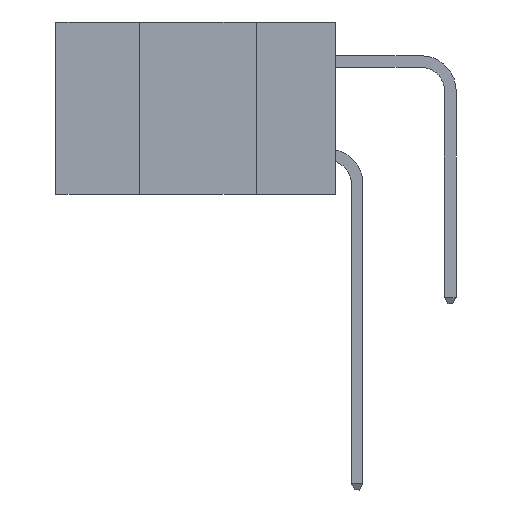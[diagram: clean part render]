
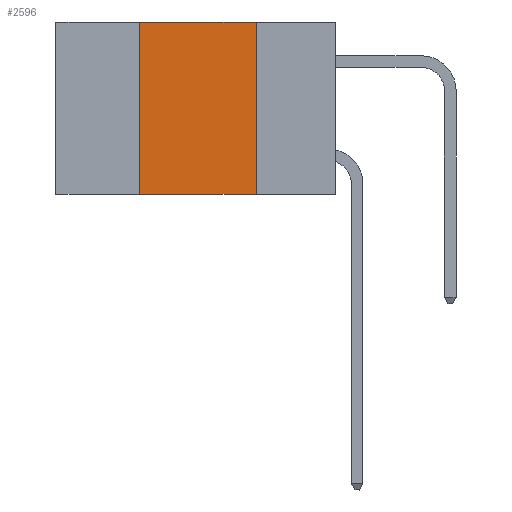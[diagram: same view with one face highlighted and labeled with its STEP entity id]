
A CAD part, left-side view. The second image highlights one B-rep face of the part: STEP entity #2596.
In plain terms, the highlighted planar face has unit normal (-1, 0, 0).
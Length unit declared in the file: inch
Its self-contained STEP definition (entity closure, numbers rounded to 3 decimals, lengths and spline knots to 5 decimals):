
#78 = ORIENTED_EDGE ( 'NONE', *, *, #10042, .F. ) ;
#564 = DIRECTION ( 'NONE',  ( 0., 0., -1. ) ) ;
#1572 = FACE_OUTER_BOUND ( 'NONE', #10146, .T. ) ;
#1748 = VECTOR ( 'NONE', #9072, 39.37008 ) ;
#2490 = VERTEX_POINT ( 'NONE', #11880 ) ;
#2596 = ADVANCED_FACE ( 'NONE', ( #1572 ), #7301, .F. ) ;
#2617 = CARTESIAN_POINT ( 'NONE',  ( 0., 0.17, 0. ) ) ;
#2675 = DIRECTION ( 'NONE',  ( 0., 0., -1. ) ) ;
#2795 = VECTOR ( 'NONE', #2675, 39.37008 ) ;
#2965 = CARTESIAN_POINT ( 'NONE',  ( 0., 0.17, -0.37 ) ) ;
#3417 = VERTEX_POINT ( 'NONE', #8843 ) ;
#3443 = CARTESIAN_POINT ( 'NONE',  ( 0., 0.6, -0.37 ) ) ;
#4071 = ORIENTED_EDGE ( 'NONE', *, *, #11199, .T. ) ;
#4833 = ORIENTED_EDGE ( 'NONE', *, *, #7839, .F. ) ;
#5103 = DIRECTION ( 'NONE',  ( 0., 0., 1. ) ) ;
#7301 = PLANE ( 'NONE',  #7825 ) ;
#7598 = EDGE_CURVE ( 'NONE', #2490, #3417, #8011, .T. ) ;
#7825 = AXIS2_PLACEMENT_3D ( 'NONE', #8306, #9355, #564 ) ;
#7839 = EDGE_CURVE ( 'NONE', #10938, #2490, #11617, .T. ) ;
#8011 = LINE ( 'NONE', #9011, #1748 ) ;
#8306 = CARTESIAN_POINT ( 'NONE',  ( 0., 0.6, 0. ) ) ;
#8341 = DIRECTION ( 'NONE',  ( 0., -1., 0. ) ) ;
#8643 = LINE ( 'NONE', #2617, #2795 ) ;
#8767 = VECTOR ( 'NONE', #8341, 39.37008 ) ;
#8843 = CARTESIAN_POINT ( 'NONE',  ( 0., 0.17, 0. ) ) ;
#9011 = CARTESIAN_POINT ( 'NONE',  ( 0., 0.6, 0. ) ) ;
#9072 = DIRECTION ( 'NONE',  ( 0., -1., 0. ) ) ;
#9355 = DIRECTION ( 'NONE',  ( 1., 0., 0. ) ) ;
#10042 = EDGE_CURVE ( 'NONE', #3417, #10631, #8643, .T. ) ;
#10146 = EDGE_LOOP ( 'NONE', ( #78, #10840, #4833, #4071 ) ) ;
#10631 = VERTEX_POINT ( 'NONE', #2965 ) ;
#10840 = ORIENTED_EDGE ( 'NONE', *, *, #7598, .F. ) ;
#10938 = VERTEX_POINT ( 'NONE', #11415 ) ;
#11199 = EDGE_CURVE ( 'NONE', #10938, #10631, #12168, .T. ) ;
#11415 = CARTESIAN_POINT ( 'NONE',  ( 0., 0.42, -0.37 ) ) ;
#11552 = CARTESIAN_POINT ( 'NONE',  ( 0., 0.42, 0. ) ) ;
#11617 = LINE ( 'NONE', #11552, #12170 ) ;
#11880 = CARTESIAN_POINT ( 'NONE',  ( 0., 0.42, 0. ) ) ;
#12168 = LINE ( 'NONE', #3443, #8767 ) ;
#12170 = VECTOR ( 'NONE', #5103, 39.37008 ) ;
